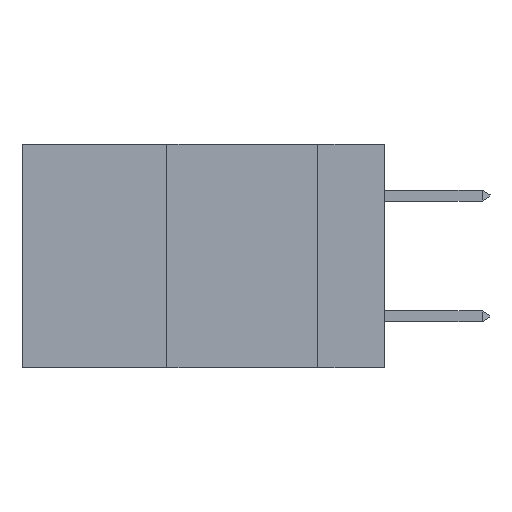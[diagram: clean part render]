
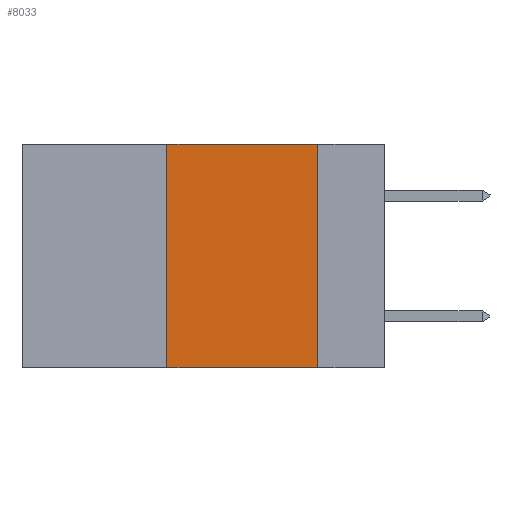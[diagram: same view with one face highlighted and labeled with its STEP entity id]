
A CAD part, left-side view. The second image highlights one B-rep face of the part: STEP entity #8033.
In plain terms, the highlighted planar face has unit normal (-1, 0, 0).
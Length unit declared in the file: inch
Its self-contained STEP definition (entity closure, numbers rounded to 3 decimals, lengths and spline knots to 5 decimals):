
#990 = VERTEX_POINT ( 'NONE', #6875 ) ;
#1680 = CARTESIAN_POINT ( 'NONE',  ( 0., 0.6, 0. ) ) ;
#1743 = CARTESIAN_POINT ( 'NONE',  ( 0., 0.36, 0. ) ) ;
#2144 = FACE_OUTER_BOUND ( 'NONE', #14343, .T. ) ;
#4264 = AXIS2_PLACEMENT_3D ( 'NONE', #1680, #27514, #8314 ) ;
#4710 = LINE ( 'NONE', #15697, #8477 ) ;
#5699 = LINE ( 'NONE', #18371, #15220 ) ;
#6264 = ORIENTED_EDGE ( 'NONE', *, *, #24873, .T. ) ;
#6731 = LINE ( 'NONE', #1743, #15913 ) ;
#6875 = CARTESIAN_POINT ( 'NONE',  ( 0., 0.36, 0. ) ) ;
#8033 = ADVANCED_FACE ( 'NONE', ( #2144 ), #25591, .F. ) ;
#8201 = DIRECTION ( 'NONE',  ( 0., -1., 0. ) ) ;
#8314 = DIRECTION ( 'NONE',  ( 0., 0., -1. ) ) ;
#8477 = VECTOR ( 'NONE', #9161, 39.37008 ) ;
#9161 = DIRECTION ( 'NONE',  ( 0., 0., -1. ) ) ;
#9498 = VERTEX_POINT ( 'NONE', #18477 ) ;
#10814 = LINE ( 'NONE', #18796, #21010 ) ;
#11110 = VERTEX_POINT ( 'NONE', #11777 ) ;
#11777 = CARTESIAN_POINT ( 'NONE',  ( 0., 0.36, -0.37 ) ) ;
#12907 = EDGE_CURVE ( 'NONE', #990, #25849, #5699, .T. ) ;
#12950 = CARTESIAN_POINT ( 'NONE',  ( 0., 0.11, 0. ) ) ;
#14343 = EDGE_LOOP ( 'NONE', ( #15428, #26696, #18206, #6264 ) ) ;
#15220 = VECTOR ( 'NONE', #16321, 39.37008 ) ;
#15428 = ORIENTED_EDGE ( 'NONE', *, *, #17376, .F. ) ;
#15697 = CARTESIAN_POINT ( 'NONE',  ( 0., 0.11, 0. ) ) ;
#15913 = VECTOR ( 'NONE', #25832, 39.37008 ) ;
#16321 = DIRECTION ( 'NONE',  ( 0., -1., 0. ) ) ;
#17376 = EDGE_CURVE ( 'NONE', #25849, #9498, #4710, .T. ) ;
#18206 = ORIENTED_EDGE ( 'NONE', *, *, #25073, .F. ) ;
#18371 = CARTESIAN_POINT ( 'NONE',  ( 0., 0.6, 0. ) ) ;
#18477 = CARTESIAN_POINT ( 'NONE',  ( 0., 0.11, -0.37 ) ) ;
#18796 = CARTESIAN_POINT ( 'NONE',  ( 0., 0.6, -0.37 ) ) ;
#21010 = VECTOR ( 'NONE', #8201, 39.37008 ) ;
#24873 = EDGE_CURVE ( 'NONE', #11110, #9498, #10814, .T. ) ;
#25073 = EDGE_CURVE ( 'NONE', #11110, #990, #6731, .T. ) ;
#25591 = PLANE ( 'NONE',  #4264 ) ;
#25832 = DIRECTION ( 'NONE',  ( 0., 0., 1. ) ) ;
#25849 = VERTEX_POINT ( 'NONE', #12950 ) ;
#26696 = ORIENTED_EDGE ( 'NONE', *, *, #12907, .F. ) ;
#27514 = DIRECTION ( 'NONE',  ( 1., 0., 0. ) ) ;
